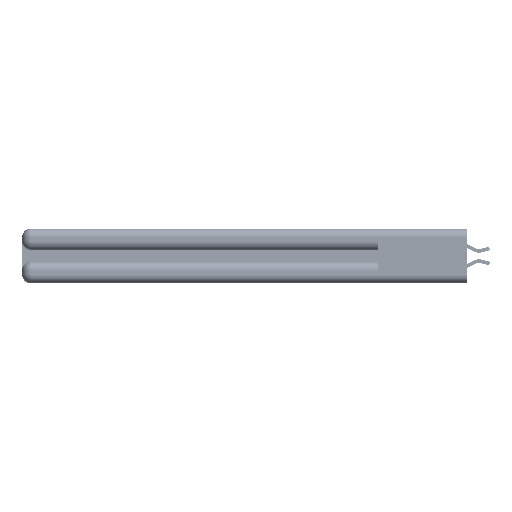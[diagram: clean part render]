
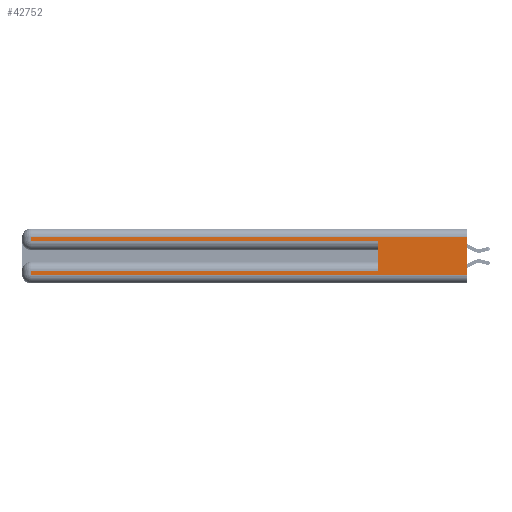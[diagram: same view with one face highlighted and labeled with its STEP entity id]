
A CAD part, left-side view. The second image highlights one B-rep face of the part: STEP entity #42752.
In plain terms, the highlighted planar face has unit normal (-1, 0, 0).
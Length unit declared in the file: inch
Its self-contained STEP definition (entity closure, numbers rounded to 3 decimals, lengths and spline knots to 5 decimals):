
#268 = DIRECTION ( 'NONE',  ( 0., 0., -1. ) ) ;
#635 = LINE ( 'NONE', #34954, #35487 ) ;
#1892 = LINE ( 'NONE', #20262, #44437 ) ;
#1925 = DIRECTION ( 'NONE',  ( 0., 0., -1. ) ) ;
#4331 = FACE_OUTER_BOUND ( 'NONE', #25959, .T. ) ;
#4626 = EDGE_CURVE ( 'NONE', #12971, #49371, #19242, .T. ) ;
#5023 = EDGE_CURVE ( 'NONE', #44225, #50485, #31474, .T. ) ;
#6054 = DIRECTION ( 'NONE',  ( 0., 1., 0. ) ) ;
#6518 = LINE ( 'NONE', #49008, #42690 ) ;
#8041 = ORIENTED_EDGE ( 'NONE', *, *, #10367, .T. ) ;
#8147 = CARTESIAN_POINT ( 'NONE',  ( 0., 0., 0.37 ) ) ;
#10094 = CARTESIAN_POINT ( 'NONE',  ( 0., 0., 0.31 ) ) ;
#10367 = EDGE_CURVE ( 'NONE', #46818, #23797, #18957, .T. ) ;
#10427 = ORIENTED_EDGE ( 'NONE', *, *, #5023, .T. ) ;
#12419 = CARTESIAN_POINT ( 'NONE',  ( 0., 2.94, 0.37 ) ) ;
#12971 = VERTEX_POINT ( 'NONE', #45398 ) ;
#13314 = EDGE_CURVE ( 'NONE', #32744, #23496, #635, .T. ) ;
#13322 = CARTESIAN_POINT ( 'NONE',  ( 0., 0., 0.085 ) ) ;
#14135 = ORIENTED_EDGE ( 'NONE', *, *, #35348, .F. ) ;
#14498 = DIRECTION ( 'NONE',  ( 0., -1., 0. ) ) ;
#16039 = VECTOR ( 'NONE', #38899, 39.37008 ) ;
#16088 = DIRECTION ( 'NONE',  ( 0., 0., 1. ) ) ;
#17678 = VECTOR ( 'NONE', #14498, 39.37008 ) ;
#18227 = CARTESIAN_POINT ( 'NONE',  ( 0., 0.6, 0.285 ) ) ;
#18290 = CARTESIAN_POINT ( 'NONE',  ( 0., 0., 0.06 ) ) ;
#18957 = LINE ( 'NONE', #18290, #17678 ) ;
#19099 = CARTESIAN_POINT ( 'NONE',  ( 0., 2.94, 0.285 ) ) ;
#19242 = LINE ( 'NONE', #13322, #16039 ) ;
#19857 = VECTOR ( 'NONE', #41627, 39.37008 ) ;
#20262 = CARTESIAN_POINT ( 'NONE',  ( 0., 0.6, 0.145 ) ) ;
#20525 = VECTOR ( 'NONE', #24912, 39.37008 ) ;
#21981 = PLANE ( 'NONE',  #41583 ) ;
#22147 = CARTESIAN_POINT ( 'NONE',  ( 0., 0., 0.37 ) ) ;
#23496 = VERTEX_POINT ( 'NONE', #39635 ) ;
#23797 = VERTEX_POINT ( 'NONE', #33499 ) ;
#24912 = DIRECTION ( 'NONE',  ( 0., -1., 0. ) ) ;
#25959 = EDGE_LOOP ( 'NONE', ( #14135, #43380, #29033, #10427, #43802, #40676, #39364, #8041 ) ) ;
#26669 = DIRECTION ( 'NONE',  ( 1., 0., 0. ) ) ;
#28336 = DIRECTION ( 'NONE',  ( 0., 0., -1. ) ) ;
#29033 = ORIENTED_EDGE ( 'NONE', *, *, #31069, .T. ) ;
#29371 = CARTESIAN_POINT ( 'NONE',  ( 0., 0., 0.285 ) ) ;
#30822 = LINE ( 'NONE', #12419, #19857 ) ;
#31069 = EDGE_CURVE ( 'NONE', #23496, #44225, #30822, .T. ) ;
#31474 = LINE ( 'NONE', #29371, #20525 ) ;
#32744 = VERTEX_POINT ( 'NONE', #10094 ) ;
#33499 = CARTESIAN_POINT ( 'NONE',  ( 0., 0., 0.06 ) ) ;
#34954 = CARTESIAN_POINT ( 'NONE',  ( 0., 0., 0.31 ) ) ;
#35348 = EDGE_CURVE ( 'NONE', #32744, #23797, #38485, .T. ) ;
#35487 = VECTOR ( 'NONE', #6054, 39.37008 ) ;
#37850 = EDGE_CURVE ( 'NONE', #49371, #46818, #6518, .T. ) ;
#38485 = LINE ( 'NONE', #8147, #39153 ) ;
#38899 = DIRECTION ( 'NONE',  ( 0., 1., 0. ) ) ;
#39153 = VECTOR ( 'NONE', #268, 39.37008 ) ;
#39364 = ORIENTED_EDGE ( 'NONE', *, *, #37850, .T. ) ;
#39635 = CARTESIAN_POINT ( 'NONE',  ( 0., 2.94, 0.31 ) ) ;
#39880 = CARTESIAN_POINT ( 'NONE',  ( 0., 2.94, 0.06 ) ) ;
#40676 = ORIENTED_EDGE ( 'NONE', *, *, #4626, .T. ) ;
#41583 = AXIS2_PLACEMENT_3D ( 'NONE', #22147, #26669, #1925 ) ;
#41627 = DIRECTION ( 'NONE',  ( 0., 0., -1. ) ) ;
#42690 = VECTOR ( 'NONE', #28336, 39.37008 ) ;
#42752 = ADVANCED_FACE ( 'NONE', ( #4331 ), #21981, .F. ) ;
#43380 = ORIENTED_EDGE ( 'NONE', *, *, #13314, .T. ) ;
#43552 = CARTESIAN_POINT ( 'NONE',  ( 0., 2.94, 0.085 ) ) ;
#43802 = ORIENTED_EDGE ( 'NONE', *, *, #51579, .F. ) ;
#44225 = VERTEX_POINT ( 'NONE', #19099 ) ;
#44437 = VECTOR ( 'NONE', #16088, 39.37008 ) ;
#45398 = CARTESIAN_POINT ( 'NONE',  ( 0., 0.6, 0.085 ) ) ;
#46818 = VERTEX_POINT ( 'NONE', #39880 ) ;
#49008 = CARTESIAN_POINT ( 'NONE',  ( 0., 2.94, 0.37 ) ) ;
#49371 = VERTEX_POINT ( 'NONE', #43552 ) ;
#50485 = VERTEX_POINT ( 'NONE', #18227 ) ;
#51579 = EDGE_CURVE ( 'NONE', #12971, #50485, #1892, .T. ) ;
